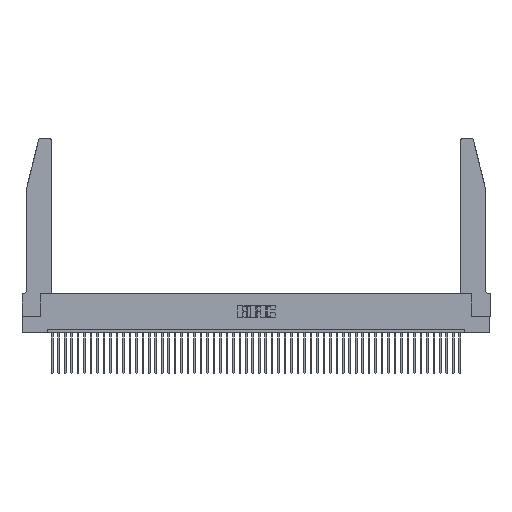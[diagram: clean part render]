
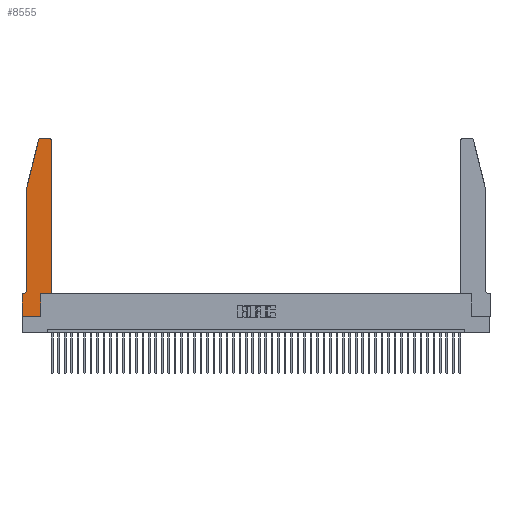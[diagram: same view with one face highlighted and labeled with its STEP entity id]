
A CAD part, top view. The second image highlights one B-rep face of the part: STEP entity #8555.
In plain terms, the highlighted planar face has unit normal (0, 0, 1).
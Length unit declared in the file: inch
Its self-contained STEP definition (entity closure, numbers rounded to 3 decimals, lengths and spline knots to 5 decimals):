
#155 = DIRECTION ( 'NONE',  ( 1., 0., 0. ) ) ;
#1291 = LINE ( 'NONE', #27206, #41128 ) ;
#2210 = ORIENTED_EDGE ( 'NONE', *, *, #48603, .T. ) ;
#2407 = DIRECTION ( 'NONE',  ( -1., 0., 0. ) ) ;
#2758 = FACE_OUTER_BOUND ( 'NONE', #38901, .T. ) ;
#3254 = ORIENTED_EDGE ( 'NONE', *, *, #5266, .T. ) ;
#3767 = CARTESIAN_POINT ( 'NONE',  ( 0., 0.35, 0.37 ) ) ;
#4591 = CARTESIAN_POINT ( 'NONE',  ( 0.4505, 2.72, 0.37 ) ) ;
#5266 = EDGE_CURVE ( 'NONE', #16611, #14516, #20193, .T. ) ;
#5448 = DIRECTION ( 'NONE',  ( 0., 0., 1. ) ) ;
#5703 = DIRECTION ( 'NONE',  ( 1., 0., 0. ) ) ;
#5775 = CIRCLE ( 'NONE', #13299, 0.03 ) ;
#7182 = ORIENTED_EDGE ( 'NONE', *, *, #18157, .T. ) ;
#7772 = VERTEX_POINT ( 'NONE', #46008 ) ;
#7951 = LINE ( 'NONE', #21505, #41730 ) ;
#8075 = CARTESIAN_POINT ( 'NONE',  ( 0.4505, 0.35, 0.37 ) ) ;
#8209 = EDGE_CURVE ( 'NONE', #46454, #30206, #26832, .T. ) ;
#8252 = DIRECTION ( 'NONE',  ( 0., -1., 0. ) ) ;
#8415 = DIRECTION ( 'NONE',  ( -1., 0., 0. ) ) ;
#8555 = ADVANCED_FACE ( 'NONE', ( #2758 ), #26448, .T. ) ;
#9291 = ORIENTED_EDGE ( 'NONE', *, *, #17709, .T. ) ;
#10760 = CARTESIAN_POINT ( 'NONE',  ( 0.4505, 0.35, 0.37 ) ) ;
#11280 = VECTOR ( 'NONE', #31850, 39.37008 ) ;
#11617 = EDGE_CURVE ( 'NONE', #23975, #47159, #25908, .T. ) ;
#11737 = DIRECTION ( 'NONE',  ( 0., 1., 0. ) ) ;
#12162 = VERTEX_POINT ( 'NONE', #24878 ) ;
#12905 = CARTESIAN_POINT ( 'NONE',  ( 0.0755, 2., 0.37 ) ) ;
#13299 = AXIS2_PLACEMENT_3D ( 'NONE', #32594, #5448, #32419 ) ;
#14280 = VECTOR ( 'NONE', #42633, 39.37008 ) ;
#14516 = VERTEX_POINT ( 'NONE', #4591 ) ;
#15523 = DIRECTION ( 'NONE',  ( 1., 0., 0. ) ) ;
#15565 = ORIENTED_EDGE ( 'NONE', *, *, #33080, .T. ) ;
#16309 = CARTESIAN_POINT ( 'NONE',  ( 0.2865, 0.35, 0.37 ) ) ;
#16611 = VERTEX_POINT ( 'NONE', #10760 ) ;
#17699 = CARTESIAN_POINT ( 'NONE',  ( 0.0755, 0.35, 0.37 ) ) ;
#17709 = EDGE_CURVE ( 'NONE', #30206, #12162, #41529, .T. ) ;
#18157 = EDGE_CURVE ( 'NONE', #7772, #16611, #34840, .T. ) ;
#19174 = CARTESIAN_POINT ( 'NONE',  ( 0.4205, 2.72, 0.37 ) ) ;
#19668 = DIRECTION ( 'NONE',  ( 0., 0., -1. ) ) ;
#20193 = LINE ( 'NONE', #48123, #27464 ) ;
#20321 = CARTESIAN_POINT ( 'NONE',  ( 0.4205, 2.75, 0.37 ) ) ;
#20465 = CARTESIAN_POINT ( 'NONE',  ( 0.0055, 0.35, 0.37 ) ) ;
#21403 = CARTESIAN_POINT ( 'NONE',  ( 0.25487, 2.72718, 0.37 ) ) ;
#21505 = CARTESIAN_POINT ( 'NONE',  ( 0., 0., 0.37 ) ) ;
#22802 = EDGE_CURVE ( 'NONE', #48453, #26119, #1291, .T. ) ;
#23975 = VERTEX_POINT ( 'NONE', #20465 ) ;
#24795 = ORIENTED_EDGE ( 'NONE', *, *, #22802, .T. ) ;
#24878 = CARTESIAN_POINT ( 'NONE',  ( 0.0755, 0.42, 0.37 ) ) ;
#25172 = EDGE_CURVE ( 'NONE', #32324, #7772, #26936, .T. ) ;
#25908 = LINE ( 'NONE', #17699, #47706 ) ;
#26119 = VERTEX_POINT ( 'NONE', #46038 ) ;
#26162 = ORIENTED_EDGE ( 'NONE', *, *, #8209, .T. ) ;
#26448 = PLANE ( 'NONE',  #34954 ) ;
#26510 = ORIENTED_EDGE ( 'NONE', *, *, #25172, .T. ) ;
#26832 = LINE ( 'NONE', #41804, #29891 ) ;
#26936 = LINE ( 'NONE', #16309, #11280 ) ;
#27206 = CARTESIAN_POINT ( 'NONE',  ( 0.2605, 2.75, 0.37 ) ) ;
#27270 = CIRCLE ( 'NONE', #47295, 0.03 ) ;
#27425 = CARTESIAN_POINT ( 'NONE',  ( 0.0055, 0.42, 0.37 ) ) ;
#27464 = VECTOR ( 'NONE', #11737, 39.37008 ) ;
#27567 = VECTOR ( 'NONE', #32496, 39.37008 ) ;
#28231 = ORIENTED_EDGE ( 'NONE', *, *, #11617, .T. ) ;
#29267 = ORIENTED_EDGE ( 'NONE', *, *, #46368, .T. ) ;
#29801 = DIRECTION ( 'NONE',  ( -0.239, -0.971, 0. ) ) ;
#29833 = LINE ( 'NONE', #31523, #30451 ) ;
#29891 = VECTOR ( 'NONE', #29801, 39.37008 ) ;
#30206 = VERTEX_POINT ( 'NONE', #39700 ) ;
#30451 = VECTOR ( 'NONE', #8252, 39.37008 ) ;
#30778 = CARTESIAN_POINT ( 'NONE',  ( 0., 0.35, 0.37 ) ) ;
#31523 = CARTESIAN_POINT ( 'NONE',  ( 0., 0., 0.37 ) ) ;
#31850 = DIRECTION ( 'NONE',  ( 0., 1., 0. ) ) ;
#32324 = VERTEX_POINT ( 'NONE', #48975 ) ;
#32419 = DIRECTION ( 'NONE',  ( 1., 0., 0. ) ) ;
#32496 = DIRECTION ( 'NONE',  ( 0., -1., 0. ) ) ;
#32594 = CARTESIAN_POINT ( 'NONE',  ( 0.284, 2.72, 0.37 ) ) ;
#32727 = VERTEX_POINT ( 'NONE', #43697 ) ;
#33080 = EDGE_CURVE ( 'NONE', #14516, #48453, #27270, .T. ) ;
#33084 = ORIENTED_EDGE ( 'NONE', *, *, #46649, .T. ) ;
#34840 = LINE ( 'NONE', #8075, #14280 ) ;
#34954 = AXIS2_PLACEMENT_3D ( 'NONE', #3767, #42030, #15523 ) ;
#38514 = CIRCLE ( 'NONE', #43872, 0.07 ) ;
#38901 = EDGE_LOOP ( 'NONE', ( #24795, #29267, #26162, #9291, #43790, #28231, #33084, #2210, #26510, #7182, #3254, #15565 ) ) ;
#39700 = CARTESIAN_POINT ( 'NONE',  ( 0.0755, 2., 0.37 ) ) ;
#41128 = VECTOR ( 'NONE', #42600, 39.37008 ) ;
#41529 = LINE ( 'NONE', #12905, #27567 ) ;
#41567 = EDGE_CURVE ( 'NONE', #12162, #23975, #38514, .T. ) ;
#41730 = VECTOR ( 'NONE', #5703, 39.37008 ) ;
#41804 = CARTESIAN_POINT ( 'NONE',  ( 0.0755, 2., 0.37 ) ) ;
#42030 = DIRECTION ( 'NONE',  ( 0., 0., 1. ) ) ;
#42600 = DIRECTION ( 'NONE',  ( -1., 0., 0. ) ) ;
#42633 = DIRECTION ( 'NONE',  ( 1., 0., 0. ) ) ;
#42815 = DIRECTION ( 'NONE',  ( 0., 0., 1. ) ) ;
#43697 = CARTESIAN_POINT ( 'NONE',  ( 0., 0., 0.37 ) ) ;
#43790 = ORIENTED_EDGE ( 'NONE', *, *, #41567, .T. ) ;
#43872 = AXIS2_PLACEMENT_3D ( 'NONE', #27425, #19668, #8415 ) ;
#46008 = CARTESIAN_POINT ( 'NONE',  ( 0.2865, 0.35, 0.37 ) ) ;
#46038 = CARTESIAN_POINT ( 'NONE',  ( 0.284, 2.75, 0.37 ) ) ;
#46368 = EDGE_CURVE ( 'NONE', #26119, #46454, #5775, .T. ) ;
#46454 = VERTEX_POINT ( 'NONE', #21403 ) ;
#46649 = EDGE_CURVE ( 'NONE', #47159, #32727, #29833, .T. ) ;
#47159 = VERTEX_POINT ( 'NONE', #30778 ) ;
#47295 = AXIS2_PLACEMENT_3D ( 'NONE', #19174, #42815, #155 ) ;
#47706 = VECTOR ( 'NONE', #2407, 39.37008 ) ;
#48123 = CARTESIAN_POINT ( 'NONE',  ( 0.4505, 0.35, 0.37 ) ) ;
#48453 = VERTEX_POINT ( 'NONE', #20321 ) ;
#48603 = EDGE_CURVE ( 'NONE', #32727, #32324, #7951, .T. ) ;
#48975 = CARTESIAN_POINT ( 'NONE',  ( 0.2865, 0., 0.37 ) ) ;
